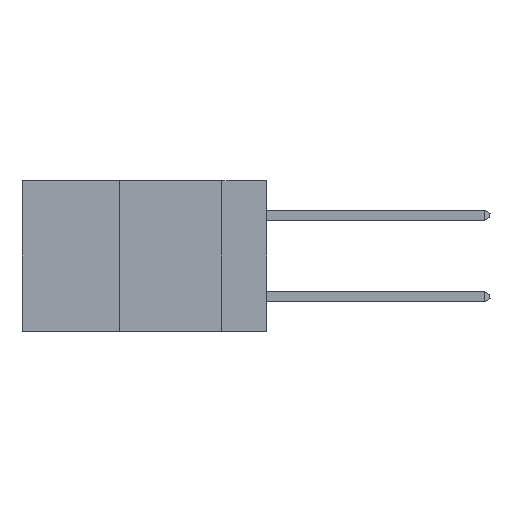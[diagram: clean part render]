
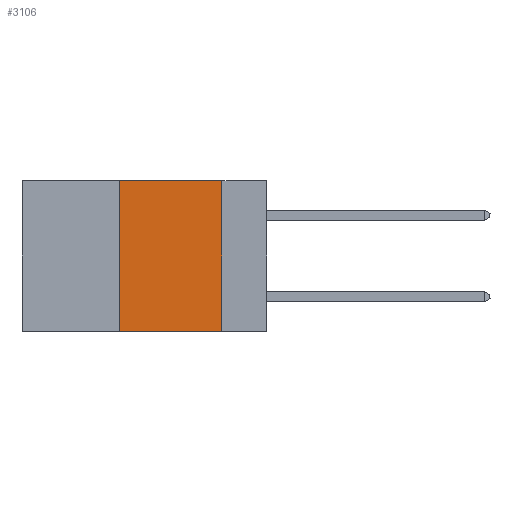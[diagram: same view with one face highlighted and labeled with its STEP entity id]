
A CAD part, left-side view. The second image highlights one B-rep face of the part: STEP entity #3106.
In plain terms, the highlighted planar face has unit normal (-1, 0, 0).
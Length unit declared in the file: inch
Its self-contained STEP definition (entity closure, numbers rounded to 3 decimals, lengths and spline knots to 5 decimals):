
#163 = CARTESIAN_POINT ( 'NONE',  ( 0., 0.11, 0. ) ) ;
#517 = CARTESIAN_POINT ( 'NONE',  ( 0., 0.6, 0. ) ) ;
#1101 = VERTEX_POINT ( 'NONE', #15048 ) ;
#1342 = CARTESIAN_POINT ( 'NONE',  ( 0., 0.36, 0. ) ) ;
#1401 = CARTESIAN_POINT ( 'NONE',  ( 0., 0.36, -0.37 ) ) ;
#3106 = ADVANCED_FACE ( 'NONE', ( #8852 ), #4329, .F. ) ;
#3326 = LINE ( 'NONE', #22370, #12391 ) ;
#3948 = VECTOR ( 'NONE', #12932, 39.37008 ) ;
#4329 = PLANE ( 'NONE',  #13913 ) ;
#4722 = CARTESIAN_POINT ( 'NONE',  ( 0., 0.11, 0. ) ) ;
#6307 = DIRECTION ( 'NONE',  ( 0., -1., 0. ) ) ;
#6763 = EDGE_CURVE ( 'NONE', #21017, #7357, #12601, .T. ) ;
#7357 = VERTEX_POINT ( 'NONE', #18949 ) ;
#7555 = EDGE_LOOP ( 'NONE', ( #14142, #14307, #14363, #14469 ) ) ;
#8036 = CARTESIAN_POINT ( 'NONE',  ( 0., 0.6, 0. ) ) ;
#8852 = FACE_OUTER_BOUND ( 'NONE', #7555, .T. ) ;
#9823 = DIRECTION ( 'NONE',  ( 0., 0., -1. ) ) ;
#12257 = DIRECTION ( 'NONE',  ( 0., 0., 1. ) ) ;
#12391 = VECTOR ( 'NONE', #6307, 39.37008 ) ;
#12601 = LINE ( 'NONE', #1342, #22018 ) ;
#12662 = VERTEX_POINT ( 'NONE', #4722 ) ;
#12932 = DIRECTION ( 'NONE',  ( 0., 0., -1. ) ) ;
#13913 = AXIS2_PLACEMENT_3D ( 'NONE', #8036, #20474, #9823 ) ;
#14142 = ORIENTED_EDGE ( 'NONE', *, *, #19922, .F. ) ;
#14307 = ORIENTED_EDGE ( 'NONE', *, *, #22541, .F. ) ;
#14363 = ORIENTED_EDGE ( 'NONE', *, *, #6763, .F. ) ;
#14469 = ORIENTED_EDGE ( 'NONE', *, *, #20791, .T. ) ;
#15048 = CARTESIAN_POINT ( 'NONE',  ( 0., 0.11, -0.37 ) ) ;
#18490 = VECTOR ( 'NONE', #22083, 39.37008 ) ;
#18949 = CARTESIAN_POINT ( 'NONE',  ( 0., 0.36, 0. ) ) ;
#19922 = EDGE_CURVE ( 'NONE', #12662, #1101, #22945, .T. ) ;
#20474 = DIRECTION ( 'NONE',  ( 1., 0., 0. ) ) ;
#20791 = EDGE_CURVE ( 'NONE', #21017, #1101, #3326, .T. ) ;
#21017 = VERTEX_POINT ( 'NONE', #1401 ) ;
#22018 = VECTOR ( 'NONE', #12257, 39.37008 ) ;
#22083 = DIRECTION ( 'NONE',  ( 0., -1., 0. ) ) ;
#22370 = CARTESIAN_POINT ( 'NONE',  ( 0., 0.6, -0.37 ) ) ;
#22541 = EDGE_CURVE ( 'NONE', #7357, #12662, #23114, .T. ) ;
#22945 = LINE ( 'NONE', #163, #3948 ) ;
#23114 = LINE ( 'NONE', #517, #18490 ) ;
